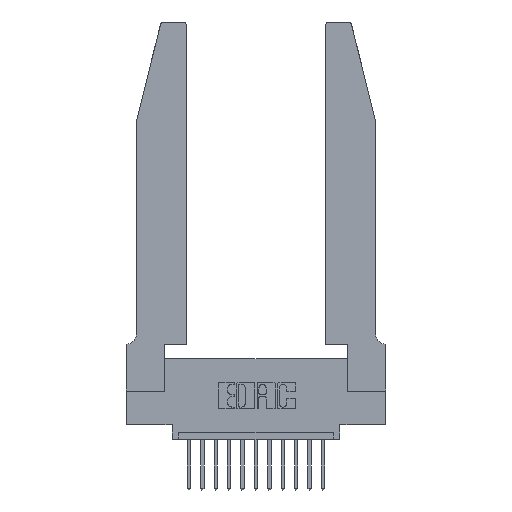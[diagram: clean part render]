
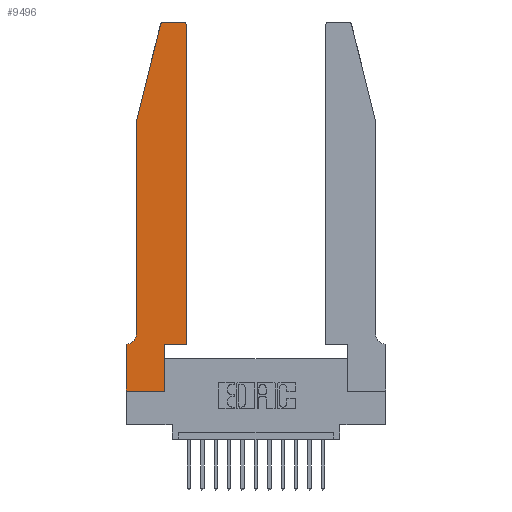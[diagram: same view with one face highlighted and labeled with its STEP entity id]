
A CAD part, top view. The second image highlights one B-rep face of the part: STEP entity #9496.
In plain terms, the highlighted planar face has unit normal (0, 0, 1).
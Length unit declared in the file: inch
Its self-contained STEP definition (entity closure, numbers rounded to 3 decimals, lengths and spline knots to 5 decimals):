
#56 = DIRECTION ( 'NONE',  ( 0., -1., 0. ) ) ;
#102 = ORIENTED_EDGE ( 'NONE', *, *, #6118, .T. ) ;
#464 = EDGE_CURVE ( 'NONE', #2198, #16256, #9283, .T. ) ;
#685 = DIRECTION ( 'NONE',  ( 0., 0., 1. ) ) ;
#869 = CARTESIAN_POINT ( 'NONE',  ( 0., 0.35, 0.37 ) ) ;
#925 = VERTEX_POINT ( 'NONE', #14222 ) ;
#1105 = CARTESIAN_POINT ( 'NONE',  ( 0.0755, 2., 0.37 ) ) ;
#1111 = VECTOR ( 'NONE', #15472, 39.37008 ) ;
#1478 = CARTESIAN_POINT ( 'NONE',  ( 0.0055, 0.42, 0.37 ) ) ;
#1697 = VECTOR ( 'NONE', #56, 39.37008 ) ;
#1989 = CARTESIAN_POINT ( 'NONE',  ( 0.2865, 0., 0.37 ) ) ;
#2008 = VERTEX_POINT ( 'NONE', #1989 ) ;
#2069 = VECTOR ( 'NONE', #11062, 39.37008 ) ;
#2198 = VERTEX_POINT ( 'NONE', #5983 ) ;
#2232 = CIRCLE ( 'NONE', #6461, 0.03 ) ;
#2375 = LINE ( 'NONE', #11642, #3217 ) ;
#2573 = CARTESIAN_POINT ( 'NONE',  ( 0.2605, 2.75, 0.37 ) ) ;
#2891 = VECTOR ( 'NONE', #8672, 39.37008 ) ;
#3054 = CARTESIAN_POINT ( 'NONE',  ( 0.4505, 0.35, 0.37 ) ) ;
#3217 = VECTOR ( 'NONE', #7715, 39.37008 ) ;
#3260 = ORIENTED_EDGE ( 'NONE', *, *, #6544, .T. ) ;
#3907 = EDGE_CURVE ( 'NONE', #4713, #2198, #9567, .T. ) ;
#3932 = VECTOR ( 'NONE', #16404, 39.37008 ) ;
#4249 = ORIENTED_EDGE ( 'NONE', *, *, #15077, .T. ) ;
#4485 = AXIS2_PLACEMENT_3D ( 'NONE', #16920, #8909, #14280 ) ;
#4548 = CARTESIAN_POINT ( 'NONE',  ( 0.4205, 2.72, 0.37 ) ) ;
#4699 = ORIENTED_EDGE ( 'NONE', *, *, #14511, .T. ) ;
#4713 = VERTEX_POINT ( 'NONE', #10127 ) ;
#4732 = DIRECTION ( 'NONE',  ( 1., 0., 0. ) ) ;
#4816 = CARTESIAN_POINT ( 'NONE',  ( 0.4505, 0.35, 0.37 ) ) ;
#5040 = AXIS2_PLACEMENT_3D ( 'NONE', #1478, #6897, #16266 ) ;
#5225 = LINE ( 'NONE', #12303, #2069 ) ;
#5290 = LINE ( 'NONE', #8235, #1697 ) ;
#5983 = CARTESIAN_POINT ( 'NONE',  ( 0.0755, 2., 0.37 ) ) ;
#6093 = AXIS2_PLACEMENT_3D ( 'NONE', #869, #685, #10251 ) ;
#6118 = EDGE_CURVE ( 'NONE', #7497, #4713, #11097, .T. ) ;
#6145 = EDGE_CURVE ( 'NONE', #16256, #14389, #15271, .T. ) ;
#6322 = VERTEX_POINT ( 'NONE', #10230 ) ;
#6459 = EDGE_CURVE ( 'NONE', #12729, #2008, #5225, .T. ) ;
#6461 = AXIS2_PLACEMENT_3D ( 'NONE', #4548, #7360, #4732 ) ;
#6519 = ORIENTED_EDGE ( 'NONE', *, *, #464, .T. ) ;
#6544 = EDGE_CURVE ( 'NONE', #8866, #925, #8805, .T. ) ;
#6897 = DIRECTION ( 'NONE',  ( 0., 0., -1. ) ) ;
#7360 = DIRECTION ( 'NONE',  ( 0., 0., 1. ) ) ;
#7373 = CARTESIAN_POINT ( 'NONE',  ( 0.0055, 0.35, 0.37 ) ) ;
#7458 = FACE_OUTER_BOUND ( 'NONE', #12740, .T. ) ;
#7497 = VERTEX_POINT ( 'NONE', #9157 ) ;
#7715 = DIRECTION ( 'NONE',  ( -1., 0., 0. ) ) ;
#7746 = EDGE_CURVE ( 'NONE', #2008, #13808, #13572, .T. ) ;
#7751 = ORIENTED_EDGE ( 'NONE', *, *, #7746, .T. ) ;
#7859 = ORIENTED_EDGE ( 'NONE', *, *, #6145, .T. ) ;
#8029 = ORIENTED_EDGE ( 'NONE', *, *, #15752, .T. ) ;
#8154 = CARTESIAN_POINT ( 'NONE',  ( 0.4205, 2.75, 0.37 ) ) ;
#8235 = CARTESIAN_POINT ( 'NONE',  ( 0., 0., 0.37 ) ) ;
#8672 = DIRECTION ( 'NONE',  ( 0., 1., 0. ) ) ;
#8747 = CARTESIAN_POINT ( 'NONE',  ( 0.4505, 0.35, 0.37 ) ) ;
#8805 = LINE ( 'NONE', #4816, #2891 ) ;
#8866 = VERTEX_POINT ( 'NONE', #3054 ) ;
#8909 = DIRECTION ( 'NONE',  ( 0., 0., 1. ) ) ;
#8913 = ORIENTED_EDGE ( 'NONE', *, *, #9670, .T. ) ;
#8917 = PLANE ( 'NONE',  #6093 ) ;
#9076 = ORIENTED_EDGE ( 'NONE', *, *, #6459, .T. ) ;
#9139 = DIRECTION ( 'NONE',  ( -0.239, -0.971, 0. ) ) ;
#9157 = CARTESIAN_POINT ( 'NONE',  ( 0.284, 2.75, 0.37 ) ) ;
#9176 = CARTESIAN_POINT ( 'NONE',  ( 0.2865, 0.35, 0.37 ) ) ;
#9283 = LINE ( 'NONE', #11106, #16002 ) ;
#9496 = ADVANCED_FACE ( 'NONE', ( #7458 ), #8917, .T. ) ;
#9567 = LINE ( 'NONE', #1105, #17311 ) ;
#9670 = EDGE_CURVE ( 'NONE', #14389, #6322, #2375, .T. ) ;
#10127 = CARTESIAN_POINT ( 'NONE',  ( 0.25487, 2.72718, 0.37 ) ) ;
#10230 = CARTESIAN_POINT ( 'NONE',  ( 0., 0.35, 0.37 ) ) ;
#10251 = DIRECTION ( 'NONE',  ( 1., 0., 0. ) ) ;
#10345 = LINE ( 'NONE', #8747, #1111 ) ;
#10842 = CARTESIAN_POINT ( 'NONE',  ( 0.2865, 0.35, 0.37 ) ) ;
#11062 = DIRECTION ( 'NONE',  ( 1., 0., 0. ) ) ;
#11097 = CIRCLE ( 'NONE', #4485, 0.03 ) ;
#11106 = CARTESIAN_POINT ( 'NONE',  ( 0.0755, 2., 0.37 ) ) ;
#11642 = CARTESIAN_POINT ( 'NONE',  ( 0.0755, 0.35, 0.37 ) ) ;
#12303 = CARTESIAN_POINT ( 'NONE',  ( 0., 0., 0.37 ) ) ;
#12525 = ORIENTED_EDGE ( 'NONE', *, *, #12586, .T. ) ;
#12586 = EDGE_CURVE ( 'NONE', #925, #17114, #2232, .T. ) ;
#12627 = DIRECTION ( 'NONE',  ( 0., -1., 0. ) ) ;
#12729 = VERTEX_POINT ( 'NONE', #16820 ) ;
#12740 = EDGE_LOOP ( 'NONE', ( #4699, #102, #16968, #6519, #7859, #8913, #8029, #9076, #7751, #4249, #3260, #12525 ) ) ;
#13249 = CARTESIAN_POINT ( 'NONE',  ( 0.0755, 0.42, 0.37 ) ) ;
#13299 = VECTOR ( 'NONE', #17229, 39.37008 ) ;
#13572 = LINE ( 'NONE', #10842, #3932 ) ;
#13808 = VERTEX_POINT ( 'NONE', #9176 ) ;
#14222 = CARTESIAN_POINT ( 'NONE',  ( 0.4505, 2.72, 0.37 ) ) ;
#14280 = DIRECTION ( 'NONE',  ( 1., 0., 0. ) ) ;
#14389 = VERTEX_POINT ( 'NONE', #7373 ) ;
#14511 = EDGE_CURVE ( 'NONE', #17114, #7497, #15178, .T. ) ;
#15077 = EDGE_CURVE ( 'NONE', #13808, #8866, #10345, .T. ) ;
#15178 = LINE ( 'NONE', #2573, #13299 ) ;
#15271 = CIRCLE ( 'NONE', #5040, 0.07 ) ;
#15472 = DIRECTION ( 'NONE',  ( 1., 0., 0. ) ) ;
#15752 = EDGE_CURVE ( 'NONE', #6322, #12729, #5290, .T. ) ;
#16002 = VECTOR ( 'NONE', #12627, 39.37008 ) ;
#16256 = VERTEX_POINT ( 'NONE', #13249 ) ;
#16266 = DIRECTION ( 'NONE',  ( -1., 0., 0. ) ) ;
#16404 = DIRECTION ( 'NONE',  ( 0., 1., 0. ) ) ;
#16820 = CARTESIAN_POINT ( 'NONE',  ( 0., 0., 0.37 ) ) ;
#16920 = CARTESIAN_POINT ( 'NONE',  ( 0.284, 2.72, 0.37 ) ) ;
#16968 = ORIENTED_EDGE ( 'NONE', *, *, #3907, .T. ) ;
#17114 = VERTEX_POINT ( 'NONE', #8154 ) ;
#17229 = DIRECTION ( 'NONE',  ( -1., 0., 0. ) ) ;
#17311 = VECTOR ( 'NONE', #9139, 39.37008 ) ;
